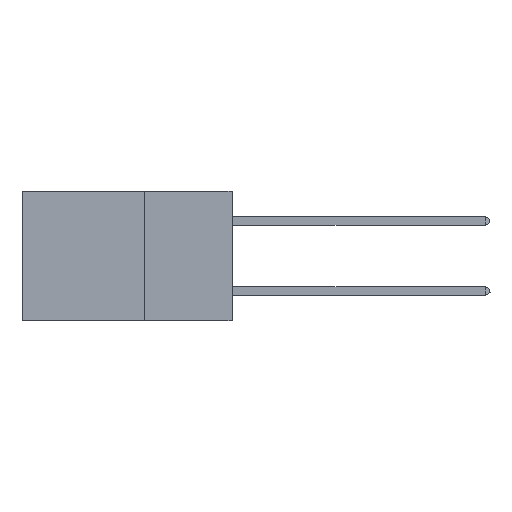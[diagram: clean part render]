
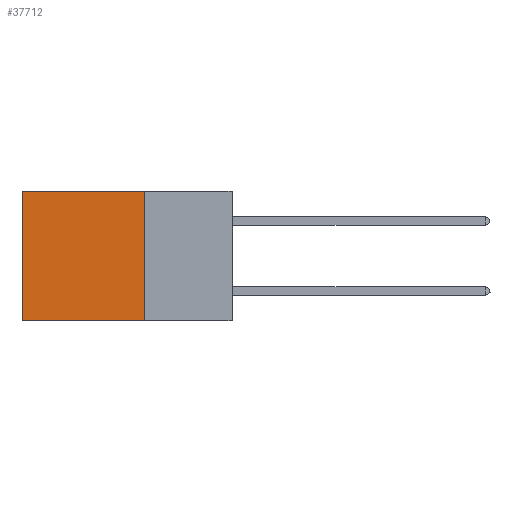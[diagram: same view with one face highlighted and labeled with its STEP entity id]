
A CAD part, left-side view. The second image highlights one B-rep face of the part: STEP entity #37712.
In plain terms, the highlighted planar face has unit normal (-1, 0, 0).
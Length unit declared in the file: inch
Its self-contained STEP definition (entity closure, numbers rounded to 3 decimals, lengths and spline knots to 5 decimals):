
#517 = DIRECTION ( 'NONE',  ( 0., 1., 0. ) ) ;
#861 = PLANE ( 'NONE',  #14994 ) ;
#1110 = VERTEX_POINT ( 'NONE', #39308 ) ;
#1554 = CARTESIAN_POINT ( 'NONE',  ( 0.2875, 0.25, -0.37 ) ) ;
#2307 = DIRECTION ( 'NONE',  ( 0., 0., -1. ) ) ;
#3129 = CARTESIAN_POINT ( 'NONE',  ( 0.2875, 0.6, -0.37 ) ) ;
#5693 = LINE ( 'NONE', #31661, #22861 ) ;
#6076 = VERTEX_POINT ( 'NONE', #11289 ) ;
#7273 = CARTESIAN_POINT ( 'NONE',  ( 0.2875, 0.25, 0. ) ) ;
#10263 = LINE ( 'NONE', #19797, #11253 ) ;
#10563 = DIRECTION ( 'NONE',  ( 0., 0., -1. ) ) ;
#11253 = VECTOR ( 'NONE', #39004, 39.37008 ) ;
#11289 = CARTESIAN_POINT ( 'NONE',  ( 0.2875, 0.25, 0. ) ) ;
#12514 = EDGE_CURVE ( 'NONE', #6076, #1110, #38989, .T. ) ;
#14994 = AXIS2_PLACEMENT_3D ( 'NONE', #7273, #22794, #10563 ) ;
#17629 = CARTESIAN_POINT ( 'NONE',  ( 0.2875, 0.6, 0. ) ) ;
#18959 = VECTOR ( 'NONE', #29284, 39.37008 ) ;
#19797 = CARTESIAN_POINT ( 'NONE',  ( 0.2875, 0.6, 0. ) ) ;
#20371 = VERTEX_POINT ( 'NONE', #17629 ) ;
#21182 = EDGE_LOOP ( 'NONE', ( #24595, #26193, #25047, #37171 ) ) ;
#21632 = CARTESIAN_POINT ( 'NONE',  ( 0.2875, 0.25, 0. ) ) ;
#22413 = LINE ( 'NONE', #1554, #18959 ) ;
#22794 = DIRECTION ( 'NONE',  ( 1., 0., 0. ) ) ;
#22861 = VECTOR ( 'NONE', #517, 39.37008 ) ;
#23287 = VECTOR ( 'NONE', #2307, 39.37008 ) ;
#24595 = ORIENTED_EDGE ( 'NONE', *, *, #37134, .T. ) ;
#24618 = EDGE_CURVE ( 'NONE', #6076, #20371, #5693, .T. ) ;
#25047 = ORIENTED_EDGE ( 'NONE', *, *, #12514, .F. ) ;
#26193 = ORIENTED_EDGE ( 'NONE', *, *, #39447, .F. ) ;
#29284 = DIRECTION ( 'NONE',  ( 0., 1., 0. ) ) ;
#31661 = CARTESIAN_POINT ( 'NONE',  ( 0.2875, 0.25, 0. ) ) ;
#32334 = FACE_OUTER_BOUND ( 'NONE', #21182, .T. ) ;
#37134 = EDGE_CURVE ( 'NONE', #20371, #38135, #10263, .T. ) ;
#37171 = ORIENTED_EDGE ( 'NONE', *, *, #24618, .T. ) ;
#37712 = ADVANCED_FACE ( 'NONE', ( #32334 ), #861, .F. ) ;
#38135 = VERTEX_POINT ( 'NONE', #3129 ) ;
#38989 = LINE ( 'NONE', #21632, #23287 ) ;
#39004 = DIRECTION ( 'NONE',  ( 0., 0., -1. ) ) ;
#39308 = CARTESIAN_POINT ( 'NONE',  ( 0.2875, 0.25, -0.37 ) ) ;
#39447 = EDGE_CURVE ( 'NONE', #1110, #38135, #22413, .T. ) ;
